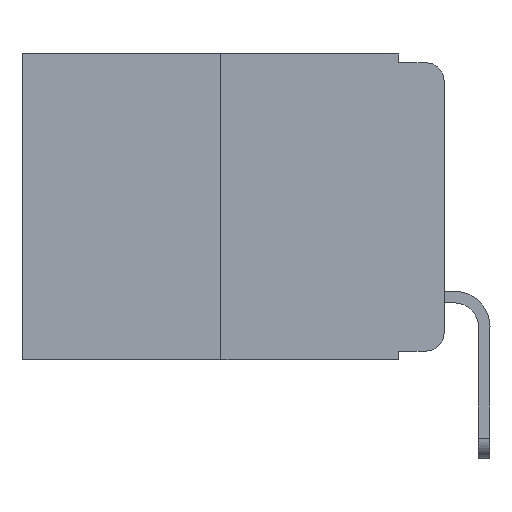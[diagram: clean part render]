
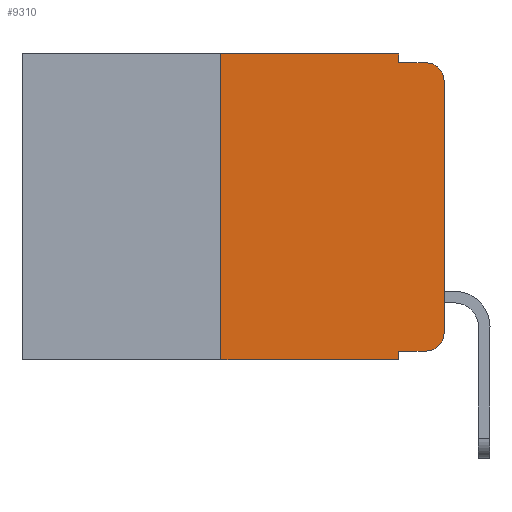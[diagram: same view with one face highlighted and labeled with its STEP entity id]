
A CAD part, left-side view. The second image highlights one B-rep face of the part: STEP entity #9310.
In plain terms, the highlighted planar face has unit normal (-1, 0, 0).
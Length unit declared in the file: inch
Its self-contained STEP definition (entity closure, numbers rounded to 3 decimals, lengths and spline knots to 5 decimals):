
#825 = CARTESIAN_POINT ( 'NONE',  ( 0., 0., -0.313 ) ) ;
#848 = ORIENTED_EDGE ( 'NONE', *, *, #2938, .F. ) ;
#974 = VERTEX_POINT ( 'NONE', #7312 ) ;
#1068 = CARTESIAN_POINT ( 'NONE',  ( 0., 0.473, 0. ) ) ;
#1098 = DIRECTION ( 'NONE',  ( 0., 0., -1. ) ) ;
#1125 = LINE ( 'NONE', #16190, #15505 ) ;
#1334 = ORIENTED_EDGE ( 'NONE', *, *, #19165, .T. ) ;
#1398 = VECTOR ( 'NONE', #4717, 39.37008 ) ;
#1665 = LINE ( 'NONE', #21739, #18606 ) ;
#2609 = LINE ( 'NONE', #15437, #10514 ) ;
#2667 = CARTESIAN_POINT ( 'NONE',  ( 0., 0.051, -0.01 ) ) ;
#2896 = AXIS2_PLACEMENT_3D ( 'NONE', #14039, #22798, #3243 ) ;
#2902 = ORIENTED_EDGE ( 'NONE', *, *, #3816, .T. ) ;
#2938 = EDGE_CURVE ( 'NONE', #19210, #14032, #16564, .T. ) ;
#3243 = DIRECTION ( 'NONE',  ( 0., 0., -1. ) ) ;
#3319 = VERTEX_POINT ( 'NONE', #14753 ) ;
#3701 = CARTESIAN_POINT ( 'NONE',  ( 0., 0.051, -0.333 ) ) ;
#3816 = EDGE_CURVE ( 'NONE', #17146, #12934, #23059, .T. ) ;
#4581 = ORIENTED_EDGE ( 'NONE', *, *, #14866, .T. ) ;
#4717 = DIRECTION ( 'NONE',  ( 0., 0., 1. ) ) ;
#5083 = ORIENTED_EDGE ( 'NONE', *, *, #7985, .T. ) ;
#6182 = ORIENTED_EDGE ( 'NONE', *, *, #19242, .F. ) ;
#6759 = LINE ( 'NONE', #10071, #1398 ) ;
#7312 = CARTESIAN_POINT ( 'NONE',  ( 0., 0.02, -0.333 ) ) ;
#7457 = EDGE_CURVE ( 'NONE', #14032, #15612, #1125, .T. ) ;
#7732 = AXIS2_PLACEMENT_3D ( 'NONE', #19088, #15376, #1098 ) ;
#7985 = EDGE_CURVE ( 'NONE', #974, #17146, #12382, .T. ) ;
#8297 = ORIENTED_EDGE ( 'NONE', *, *, #7457, .F. ) ;
#8404 = DIRECTION ( 'NONE',  ( 0., -1., 0. ) ) ;
#8476 = EDGE_CURVE ( 'NONE', #14207, #9587, #2609, .T. ) ;
#8673 = VECTOR ( 'NONE', #18295, 39.37008 ) ;
#9310 = ADVANCED_FACE ( 'NONE', ( #11983 ), #20660, .F. ) ;
#9587 = VERTEX_POINT ( 'NONE', #18279 ) ;
#10071 = CARTESIAN_POINT ( 'NONE',  ( 0., 0.25, 0. ) ) ;
#10514 = VECTOR ( 'NONE', #8404, 39.37008 ) ;
#11232 = CARTESIAN_POINT ( 'NONE',  ( 0., 0.25, -0.343 ) ) ;
#11750 = CARTESIAN_POINT ( 'NONE',  ( 0., 0.02, -0.03 ) ) ;
#11771 = VECTOR ( 'NONE', #19058, 39.37008 ) ;
#11983 = FACE_OUTER_BOUND ( 'NONE', #12840, .T. ) ;
#12382 = CIRCLE ( 'NONE', #2896, 0.02 ) ;
#12795 = DIRECTION ( 'NONE',  ( 0., -1., 0. ) ) ;
#12840 = EDGE_LOOP ( 'NONE', ( #2902, #4581, #13835, #8297, #848, #16454, #22832, #6182, #1334, #5083 ) ) ;
#12934 = VERTEX_POINT ( 'NONE', #17824 ) ;
#13341 = DIRECTION ( 'NONE',  ( -1., 0., 0. ) ) ;
#13835 = ORIENTED_EDGE ( 'NONE', *, *, #14653, .F. ) ;
#14032 = VERTEX_POINT ( 'NONE', #23302 ) ;
#14039 = CARTESIAN_POINT ( 'NONE',  ( 0., 0.02, -0.313 ) ) ;
#14207 = VERTEX_POINT ( 'NONE', #11232 ) ;
#14477 = CARTESIAN_POINT ( 'NONE',  ( 0., 0.25, 0. ) ) ;
#14564 = CARTESIAN_POINT ( 'NONE',  ( 0., 0., 0. ) ) ;
#14653 = EDGE_CURVE ( 'NONE', #15612, #3319, #15826, .T. ) ;
#14753 = CARTESIAN_POINT ( 'NONE',  ( 0., 0.02, -0.01 ) ) ;
#14866 = EDGE_CURVE ( 'NONE', #12934, #3319, #16663, .T. ) ;
#15376 = DIRECTION ( 'NONE',  ( 1., 0., 0. ) ) ;
#15437 = CARTESIAN_POINT ( 'NONE',  ( 0., 0.473, -0.343 ) ) ;
#15505 = VECTOR ( 'NONE', #17779, 39.37008 ) ;
#15612 = VERTEX_POINT ( 'NONE', #2667 ) ;
#15826 = LINE ( 'NONE', #18325, #22595 ) ;
#16051 = LINE ( 'NONE', #19462, #19438 ) ;
#16190 = CARTESIAN_POINT ( 'NONE',  ( 0., 0.051, 0. ) ) ;
#16454 = ORIENTED_EDGE ( 'NONE', *, *, #18971, .F. ) ;
#16564 = LINE ( 'NONE', #1068, #11771 ) ;
#16663 = CIRCLE ( 'NONE', #18727, 0.02 ) ;
#17146 = VERTEX_POINT ( 'NONE', #825 ) ;
#17779 = DIRECTION ( 'NONE',  ( 0., 0., -1. ) ) ;
#17824 = CARTESIAN_POINT ( 'NONE',  ( 0., 0., -0.03 ) ) ;
#18279 = CARTESIAN_POINT ( 'NONE',  ( 0., 0.051, -0.343 ) ) ;
#18295 = DIRECTION ( 'NONE',  ( 0., 0., 1. ) ) ;
#18325 = CARTESIAN_POINT ( 'NONE',  ( 0., 0.051, -0.01 ) ) ;
#18606 = VECTOR ( 'NONE', #23376, 39.37008 ) ;
#18727 = AXIS2_PLACEMENT_3D ( 'NONE', #11750, #13341, #20678 ) ;
#18971 = EDGE_CURVE ( 'NONE', #14207, #19210, #6759, .T. ) ;
#19058 = DIRECTION ( 'NONE',  ( 0., -1., 0. ) ) ;
#19088 = CARTESIAN_POINT ( 'NONE',  ( 0., 0.473, 0. ) ) ;
#19165 = EDGE_CURVE ( 'NONE', #21948, #974, #16051, .T. ) ;
#19210 = VERTEX_POINT ( 'NONE', #14477 ) ;
#19242 = EDGE_CURVE ( 'NONE', #21948, #9587, #1665, .T. ) ;
#19438 = VECTOR ( 'NONE', #21500, 39.37008 ) ;
#19462 = CARTESIAN_POINT ( 'NONE',  ( 0., 0.051, -0.333 ) ) ;
#20660 = PLANE ( 'NONE',  #7732 ) ;
#20678 = DIRECTION ( 'NONE',  ( 0., 0., -1. ) ) ;
#21500 = DIRECTION ( 'NONE',  ( 0., -1., 0. ) ) ;
#21739 = CARTESIAN_POINT ( 'NONE',  ( 0., 0.051, 0. ) ) ;
#21948 = VERTEX_POINT ( 'NONE', #3701 ) ;
#22595 = VECTOR ( 'NONE', #12795, 39.37008 ) ;
#22798 = DIRECTION ( 'NONE',  ( -1., 0., 0. ) ) ;
#22832 = ORIENTED_EDGE ( 'NONE', *, *, #8476, .T. ) ;
#23059 = LINE ( 'NONE', #14564, #8673 ) ;
#23302 = CARTESIAN_POINT ( 'NONE',  ( 0., 0.051, 0. ) ) ;
#23376 = DIRECTION ( 'NONE',  ( 0., 0., -1. ) ) ;
